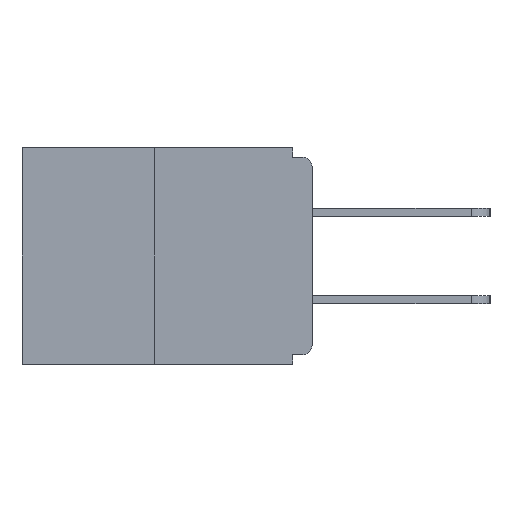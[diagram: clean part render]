
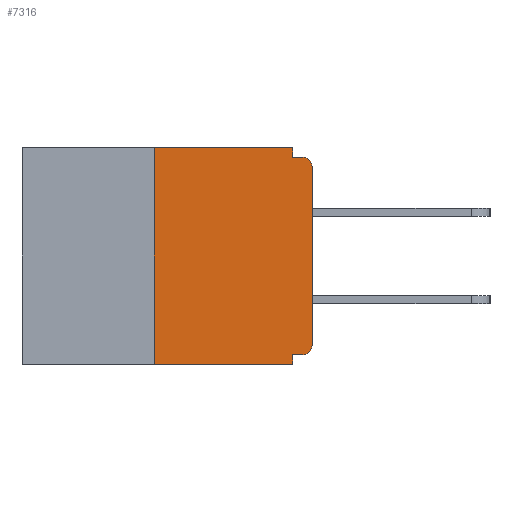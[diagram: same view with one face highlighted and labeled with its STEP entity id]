
A CAD part, left-side view. The second image highlights one B-rep face of the part: STEP entity #7316.
In plain terms, the highlighted planar face has unit normal (-1, 0, 0).
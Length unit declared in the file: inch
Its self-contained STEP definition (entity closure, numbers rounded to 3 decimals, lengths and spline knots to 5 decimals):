
#250 = VECTOR ( 'NONE', #10389, 39.37008 ) ;
#282 = VERTEX_POINT ( 'NONE', #1714 ) ;
#455 = CARTESIAN_POINT ( 'NONE',  ( 0., 0.015, -0.313 ) ) ;
#494 = EDGE_CURVE ( 'NONE', #13101, #282, #12008, .T. ) ;
#564 = DIRECTION ( 'NONE',  ( 0., 0., 1. ) ) ;
#1010 = CARTESIAN_POINT ( 'NONE',  ( 0., 0.015, -0.015 ) ) ;
#1062 = LINE ( 'NONE', #14701, #6300 ) ;
#1086 = VERTEX_POINT ( 'NONE', #8990 ) ;
#1164 = LINE ( 'NONE', #11254, #1351 ) ;
#1351 = VECTOR ( 'NONE', #564, 39.37008 ) ;
#1586 = CARTESIAN_POINT ( 'NONE',  ( 0., 0.25, 0. ) ) ;
#1714 = CARTESIAN_POINT ( 'NONE',  ( 0., 0.031, 0. ) ) ;
#1725 = ORIENTED_EDGE ( 'NONE', *, *, #9352, .T. ) ;
#1728 = CARTESIAN_POINT ( 'NONE',  ( 0., 0.031, -0.015 ) ) ;
#1753 = CARTESIAN_POINT ( 'NONE',  ( 0., 0.031, -0.343 ) ) ;
#2297 = ORIENTED_EDGE ( 'NONE', *, *, #3086, .F. ) ;
#2695 = VERTEX_POINT ( 'NONE', #1728 ) ;
#3086 = EDGE_CURVE ( 'NONE', #2695, #4190, #1062, .T. ) ;
#3203 = ORIENTED_EDGE ( 'NONE', *, *, #8400, .F. ) ;
#3832 = CARTESIAN_POINT ( 'NONE',  ( 0., 0., 0. ) ) ;
#4190 = VERTEX_POINT ( 'NONE', #1010 ) ;
#4425 = PLANE ( 'NONE',  #5936 ) ;
#4592 = ORIENTED_EDGE ( 'NONE', *, *, #5797, .F. ) ;
#4867 = ORIENTED_EDGE ( 'NONE', *, *, #8897, .F. ) ;
#4911 = CARTESIAN_POINT ( 'NONE',  ( 0., 0.031, -0.328 ) ) ;
#4917 = VERTEX_POINT ( 'NONE', #8402 ) ;
#5180 = DIRECTION ( 'NONE',  ( 0., 0., 1. ) ) ;
#5449 = DIRECTION ( 'NONE',  ( 0., 0., -1. ) ) ;
#5464 = ORIENTED_EDGE ( 'NONE', *, *, #9969, .T. ) ;
#5797 = EDGE_CURVE ( 'NONE', #11132, #10966, #8298, .T. ) ;
#5936 = AXIS2_PLACEMENT_3D ( 'NONE', #7825, #11280, #5449 ) ;
#6009 = DIRECTION ( 'NONE',  ( 0., 0., -1. ) ) ;
#6168 = DIRECTION ( 'NONE',  ( -1., 0., 0. ) ) ;
#6300 = VECTOR ( 'NONE', #12309, 39.37008 ) ;
#6599 = FACE_OUTER_BOUND ( 'NONE', #10269, .T. ) ;
#6923 = LINE ( 'NONE', #9210, #250 ) ;
#7094 = CARTESIAN_POINT ( 'NONE',  ( 0., 0.015, -0.03 ) ) ;
#7163 = AXIS2_PLACEMENT_3D ( 'NONE', #455, #6168, #9405 ) ;
#7316 = ADVANCED_FACE ( 'NONE', ( #6599 ), #4425, .F. ) ;
#7487 = CIRCLE ( 'NONE', #7163, 0.015 ) ;
#7807 = AXIS2_PLACEMENT_3D ( 'NONE', #7094, #11605, #12923 ) ;
#7825 = CARTESIAN_POINT ( 'NONE',  ( 0., 0.46, 0. ) ) ;
#7971 = CARTESIAN_POINT ( 'NONE',  ( 0., 0.46, 0. ) ) ;
#8062 = EDGE_CURVE ( 'NONE', #14372, #11132, #6923, .T. ) ;
#8298 = LINE ( 'NONE', #13171, #11016 ) ;
#8400 = EDGE_CURVE ( 'NONE', #282, #2695, #10928, .T. ) ;
#8402 = CARTESIAN_POINT ( 'NONE',  ( 0., 0., -0.03 ) ) ;
#8897 = EDGE_CURVE ( 'NONE', #10357, #13101, #1164, .T. ) ;
#8948 = VECTOR ( 'NONE', #11027, 39.37008 ) ;
#8990 = CARTESIAN_POINT ( 'NONE',  ( 0., 0., -0.313 ) ) ;
#9081 = DIRECTION ( 'NONE',  ( 0., -1., 0. ) ) ;
#9210 = CARTESIAN_POINT ( 'NONE',  ( 0., 0., -0.328 ) ) ;
#9238 = EDGE_CURVE ( 'NONE', #10357, #10966, #12531, .T. ) ;
#9249 = LINE ( 'NONE', #3832, #10359 ) ;
#9352 = EDGE_CURVE ( 'NONE', #4917, #4190, #14722, .T. ) ;
#9405 = DIRECTION ( 'NONE',  ( 0., 0., -1. ) ) ;
#9969 = EDGE_CURVE ( 'NONE', #1086, #4917, #9249, .T. ) ;
#10269 = EDGE_LOOP ( 'NONE', ( #11453, #4867, #13495, #4592, #14939, #11055, #5464, #1725, #2297, #3203 ) ) ;
#10357 = VERTEX_POINT ( 'NONE', #14321 ) ;
#10359 = VECTOR ( 'NONE', #5180, 39.37008 ) ;
#10389 = DIRECTION ( 'NONE',  ( 0., 1., 0. ) ) ;
#10626 = CARTESIAN_POINT ( 'NONE',  ( 0., 0.015, -0.328 ) ) ;
#10928 = LINE ( 'NONE', #14472, #8948 ) ;
#10966 = VERTEX_POINT ( 'NONE', #1753 ) ;
#11016 = VECTOR ( 'NONE', #6009, 39.37008 ) ;
#11027 = DIRECTION ( 'NONE',  ( 0., 0., -1. ) ) ;
#11055 = ORIENTED_EDGE ( 'NONE', *, *, #12319, .T. ) ;
#11132 = VERTEX_POINT ( 'NONE', #4911 ) ;
#11254 = CARTESIAN_POINT ( 'NONE',  ( 0., 0.25, 0. ) ) ;
#11280 = DIRECTION ( 'NONE',  ( 1., 0., 0. ) ) ;
#11453 = ORIENTED_EDGE ( 'NONE', *, *, #494, .F. ) ;
#11503 = DIRECTION ( 'NONE',  ( 0., -1., 0. ) ) ;
#11605 = DIRECTION ( 'NONE',  ( -1., 0., 0. ) ) ;
#11635 = VECTOR ( 'NONE', #11503, 39.37008 ) ;
#12008 = LINE ( 'NONE', #7971, #11635 ) ;
#12309 = DIRECTION ( 'NONE',  ( 0., -1., 0. ) ) ;
#12319 = EDGE_CURVE ( 'NONE', #14372, #1086, #7487, .T. ) ;
#12531 = LINE ( 'NONE', #12675, #13623 ) ;
#12675 = CARTESIAN_POINT ( 'NONE',  ( 0., 0.46, -0.343 ) ) ;
#12923 = DIRECTION ( 'NONE',  ( 0., 0., -1. ) ) ;
#13101 = VERTEX_POINT ( 'NONE', #1586 ) ;
#13171 = CARTESIAN_POINT ( 'NONE',  ( 0., 0.031, -0.343 ) ) ;
#13495 = ORIENTED_EDGE ( 'NONE', *, *, #9238, .T. ) ;
#13623 = VECTOR ( 'NONE', #9081, 39.37008 ) ;
#14321 = CARTESIAN_POINT ( 'NONE',  ( 0., 0.25, -0.343 ) ) ;
#14372 = VERTEX_POINT ( 'NONE', #10626 ) ;
#14472 = CARTESIAN_POINT ( 'NONE',  ( 0., 0.031, 0. ) ) ;
#14701 = CARTESIAN_POINT ( 'NONE',  ( 0., 0., -0.015 ) ) ;
#14722 = CIRCLE ( 'NONE', #7807, 0.015 ) ;
#14939 = ORIENTED_EDGE ( 'NONE', *, *, #8062, .F. ) ;
